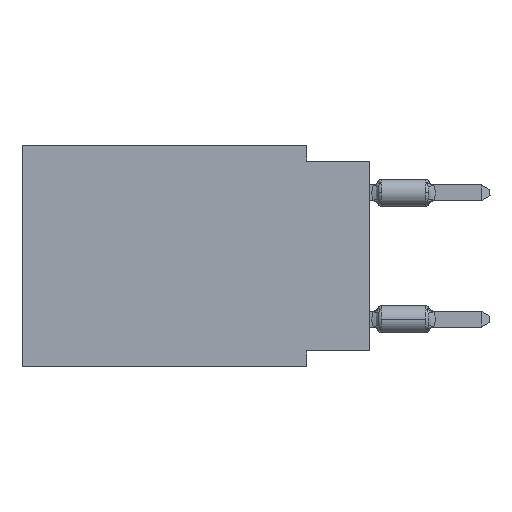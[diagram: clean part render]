
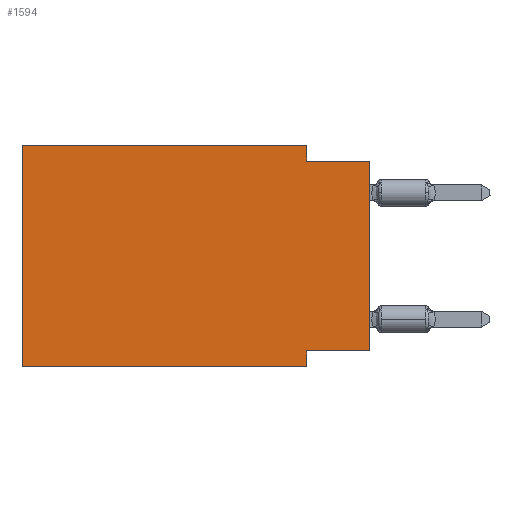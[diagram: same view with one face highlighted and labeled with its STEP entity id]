
A CAD part, left-side view. The second image highlights one B-rep face of the part: STEP entity #1594.
In plain terms, the highlighted planar face has unit normal (-1, 0, 0).
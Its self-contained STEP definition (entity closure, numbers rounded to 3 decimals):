
#486 = VECTOR ( 'NONE', #19007, 1000. ) ;
#571 = CARTESIAN_POINT ( 'NONE',  ( 0., 0., -0.635 ) ) ;
#576 = LINE ( 'NONE', #16514, #14851 ) ;
#1243 = VECTOR ( 'NONE', #9791, 1000. ) ;
#1594 = ADVANCED_FACE ( 'NONE', ( #19093 ), #23377, .F. ) ;
#1798 = LINE ( 'NONE', #9780, #7352 ) ;
#1964 = CARTESIAN_POINT ( 'NONE',  ( 0., 13.97, 0. ) ) ;
#2359 = EDGE_CURVE ( 'NONE', #3955, #17440, #3834, .T. ) ;
#3139 = CARTESIAN_POINT ( 'NONE',  ( 0., 2.54, 0. ) ) ;
#3445 = CARTESIAN_POINT ( 'NONE',  ( 0., 13.97, 0. ) ) ;
#3834 = LINE ( 'NONE', #5529, #17433 ) ;
#3871 = VECTOR ( 'NONE', #18283, 1000. ) ;
#3955 = VERTEX_POINT ( 'NONE', #13937 ) ;
#4280 = LINE ( 'NONE', #7456, #11535 ) ;
#4725 = ORIENTED_EDGE ( 'NONE', *, *, #25204, .T. ) ;
#5529 = CARTESIAN_POINT ( 'NONE',  ( 0., 2.54, -8.89 ) ) ;
#6452 = EDGE_CURVE ( 'NONE', #13791, #23319, #17178, .T. ) ;
#6589 = DIRECTION ( 'NONE',  ( 0., 1., 0. ) ) ;
#7352 = VECTOR ( 'NONE', #8060, 1000. ) ;
#7456 = CARTESIAN_POINT ( 'NONE',  ( 0., 13.97, -8.89 ) ) ;
#7640 = VECTOR ( 'NONE', #10377, 1000. ) ;
#7958 = EDGE_CURVE ( 'NONE', #22101, #24049, #14684, .T. ) ;
#8060 = DIRECTION ( 'NONE',  ( 0., 0., -1. ) ) ;
#9534 = EDGE_CURVE ( 'NONE', #23319, #17473, #25751, .T. ) ;
#9780 = CARTESIAN_POINT ( 'NONE',  ( 0., 2.54, 0. ) ) ;
#9791 = DIRECTION ( 'NONE',  ( 0., 0., 1. ) ) ;
#10377 = DIRECTION ( 'NONE',  ( 0., -1., 0. ) ) ;
#10593 = VERTEX_POINT ( 'NONE', #15087 ) ;
#10668 = CARTESIAN_POINT ( 'NONE',  ( 0., 2.54, -0.635 ) ) ;
#11042 = AXIS2_PLACEMENT_3D ( 'NONE', #19219, #15308, #15433 ) ;
#11535 = VECTOR ( 'NONE', #15439, 1000. ) ;
#11983 = ORIENTED_EDGE ( 'NONE', *, *, #24824, .T. ) ;
#12634 = ORIENTED_EDGE ( 'NONE', *, *, #18134, .F. ) ;
#13791 = VERTEX_POINT ( 'NONE', #25104 ) ;
#13937 = CARTESIAN_POINT ( 'NONE',  ( 0., 2.54, -8.255 ) ) ;
#14296 = ORIENTED_EDGE ( 'NONE', *, *, #6452, .F. ) ;
#14684 = LINE ( 'NONE', #571, #7640 ) ;
#14773 = ORIENTED_EDGE ( 'NONE', *, *, #9534, .F. ) ;
#14851 = VECTOR ( 'NONE', #6589, 1000. ) ;
#15087 = CARTESIAN_POINT ( 'NONE',  ( 0., 0., -8.255 ) ) ;
#15172 = CARTESIAN_POINT ( 'NONE',  ( 0., 2.54, -8.89 ) ) ;
#15308 = DIRECTION ( 'NONE',  ( 1., 0., 0. ) ) ;
#15433 = DIRECTION ( 'NONE',  ( 0., 0., -1. ) ) ;
#15439 = DIRECTION ( 'NONE',  ( 0., -1., 0. ) ) ;
#16514 = CARTESIAN_POINT ( 'NONE',  ( 0., 0., -8.255 ) ) ;
#16595 = CARTESIAN_POINT ( 'NONE',  ( 0., 13.97, 0. ) ) ;
#17178 = LINE ( 'NONE', #3445, #486 ) ;
#17433 = VECTOR ( 'NONE', #19781, 1000. ) ;
#17440 = VERTEX_POINT ( 'NONE', #15172 ) ;
#17473 = VERTEX_POINT ( 'NONE', #3139 ) ;
#18134 = EDGE_CURVE ( 'NONE', #10593, #3955, #576, .T. ) ;
#18283 = DIRECTION ( 'NONE',  ( 0., -1., 0. ) ) ;
#19007 = DIRECTION ( 'NONE',  ( 0., 0., 1. ) ) ;
#19093 = FACE_OUTER_BOUND ( 'NONE', #25568, .T. ) ;
#19219 = CARTESIAN_POINT ( 'NONE',  ( 0., 13.97, 0. ) ) ;
#19230 = EDGE_CURVE ( 'NONE', #17473, #22101, #1798, .T. ) ;
#19594 = CARTESIAN_POINT ( 'NONE',  ( 0., 0., 0. ) ) ;
#19721 = LINE ( 'NONE', #19594, #1243 ) ;
#19781 = DIRECTION ( 'NONE',  ( 0., 0., -1. ) ) ;
#21138 = ORIENTED_EDGE ( 'NONE', *, *, #7958, .F. ) ;
#22101 = VERTEX_POINT ( 'NONE', #10668 ) ;
#22616 = CARTESIAN_POINT ( 'NONE',  ( 0., 0., -0.635 ) ) ;
#23319 = VERTEX_POINT ( 'NONE', #16595 ) ;
#23377 = PLANE ( 'NONE',  #11042 ) ;
#24049 = VERTEX_POINT ( 'NONE', #22616 ) ;
#24383 = ORIENTED_EDGE ( 'NONE', *, *, #2359, .F. ) ;
#24509 = ORIENTED_EDGE ( 'NONE', *, *, #19230, .F. ) ;
#24824 = EDGE_CURVE ( 'NONE', #10593, #24049, #19721, .T. ) ;
#25104 = CARTESIAN_POINT ( 'NONE',  ( 0., 13.97, -8.89 ) ) ;
#25204 = EDGE_CURVE ( 'NONE', #13791, #17440, #4280, .T. ) ;
#25568 = EDGE_LOOP ( 'NONE', ( #11983, #21138, #24509, #14773, #14296, #4725, #24383, #12634 ) ) ;
#25751 = LINE ( 'NONE', #1964, #3871 ) ;
